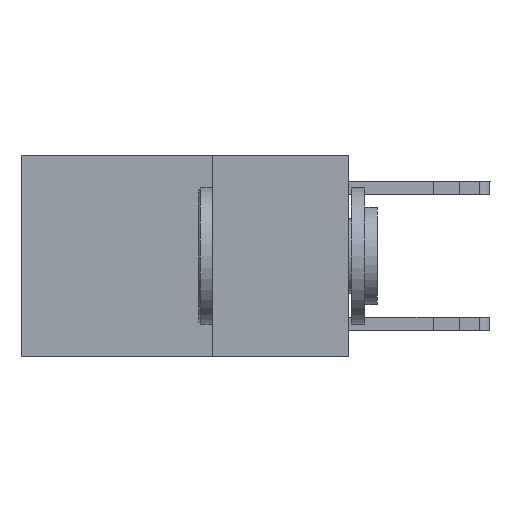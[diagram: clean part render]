
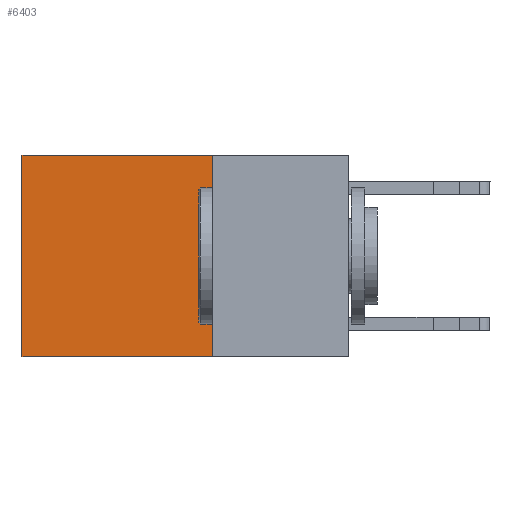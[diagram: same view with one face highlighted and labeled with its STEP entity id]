
A CAD part, left-side view. The second image highlights one B-rep face of the part: STEP entity #6403.
In plain terms, the highlighted planar face has unit normal (-1, 0, 0).
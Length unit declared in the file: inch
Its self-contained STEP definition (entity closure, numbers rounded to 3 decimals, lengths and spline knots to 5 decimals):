
#646 = ORIENTED_EDGE ( 'NONE', *, *, #15414, .T. ) ;
#1485 = CARTESIAN_POINT ( 'NONE',  ( 0.2625, 0.25, 0. ) ) ;
#1746 = ORIENTED_EDGE ( 'NONE', *, *, #13608, .F. ) ;
#2727 = CARTESIAN_POINT ( 'NONE',  ( 0.2625, 0.6, 0. ) ) ;
#3426 = VECTOR ( 'NONE', #3857, 39.37008 ) ;
#3857 = DIRECTION ( 'NONE',  ( 0., 0., -1. ) ) ;
#4923 = ORIENTED_EDGE ( 'NONE', *, *, #10359, .T. ) ;
#6222 = VERTEX_POINT ( 'NONE', #14608 ) ;
#6403 = ADVANCED_FACE ( 'NONE', ( #20688 ), #18572, .F. ) ;
#7530 = CARTESIAN_POINT ( 'NONE',  ( 0.2625, 0.25, 0. ) ) ;
#7660 = VECTOR ( 'NONE', #22377, 39.37008 ) ;
#7673 = VERTEX_POINT ( 'NONE', #24321 ) ;
#8723 = VERTEX_POINT ( 'NONE', #23190 ) ;
#9376 = AXIS2_PLACEMENT_3D ( 'NONE', #7530, #16430, #16014 ) ;
#10359 = EDGE_CURVE ( 'NONE', #8723, #26660, #24216, .T. ) ;
#11945 = ORIENTED_EDGE ( 'NONE', *, *, #12473, .F. ) ;
#12348 = DIRECTION ( 'NONE',  ( 0., 1., 0. ) ) ;
#12473 = EDGE_CURVE ( 'NONE', #7673, #26660, #15610, .T. ) ;
#13608 = EDGE_CURVE ( 'NONE', #6222, #7673, #17020, .T. ) ;
#14608 = CARTESIAN_POINT ( 'NONE',  ( 0.2625, 0.25, 0. ) ) ;
#14683 = CARTESIAN_POINT ( 'NONE',  ( 0.2625, 0.6, -0.37 ) ) ;
#14876 = CARTESIAN_POINT ( 'NONE',  ( 0.2625, 0.25, 0. ) ) ;
#15043 = CARTESIAN_POINT ( 'NONE',  ( 0.2625, 0.25, -0.37 ) ) ;
#15180 = DIRECTION ( 'NONE',  ( 0., 1., 0. ) ) ;
#15414 = EDGE_CURVE ( 'NONE', #6222, #8723, #16579, .T. ) ;
#15610 = LINE ( 'NONE', #15043, #22172 ) ;
#16014 = DIRECTION ( 'NONE',  ( 0., 0., -1. ) ) ;
#16430 = DIRECTION ( 'NONE',  ( 1., 0., 0. ) ) ;
#16579 = LINE ( 'NONE', #14876, #20709 ) ;
#17020 = LINE ( 'NONE', #1485, #3426 ) ;
#18572 = PLANE ( 'NONE',  #9376 ) ;
#20688 = FACE_OUTER_BOUND ( 'NONE', #24663, .T. ) ;
#20709 = VECTOR ( 'NONE', #12348, 39.37008 ) ;
#22172 = VECTOR ( 'NONE', #15180, 39.37008 ) ;
#22377 = DIRECTION ( 'NONE',  ( 0., 0., -1. ) ) ;
#23190 = CARTESIAN_POINT ( 'NONE',  ( 0.2625, 0.6, 0. ) ) ;
#24216 = LINE ( 'NONE', #2727, #7660 ) ;
#24321 = CARTESIAN_POINT ( 'NONE',  ( 0.2625, 0.25, -0.37 ) ) ;
#24663 = EDGE_LOOP ( 'NONE', ( #4923, #11945, #1746, #646 ) ) ;
#26660 = VERTEX_POINT ( 'NONE', #14683 ) ;
